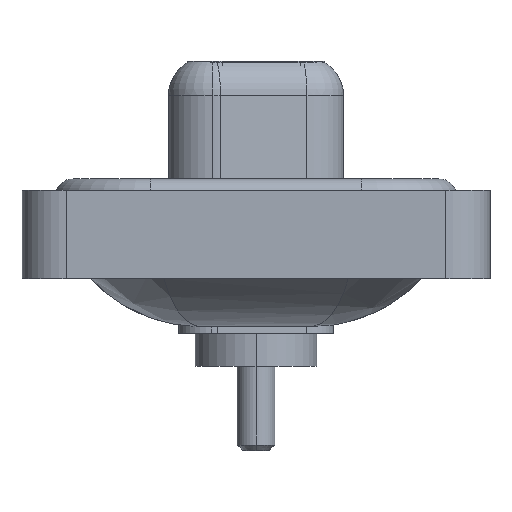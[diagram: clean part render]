
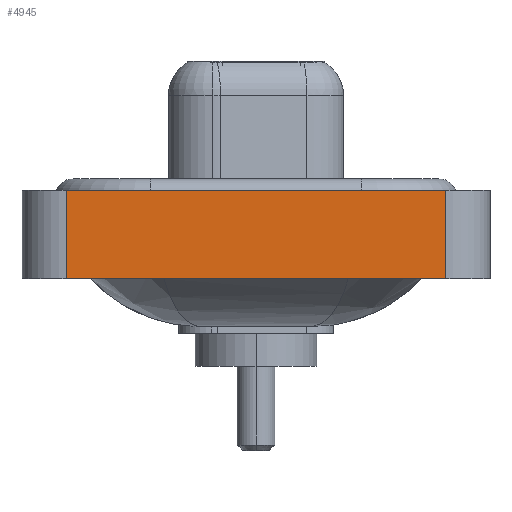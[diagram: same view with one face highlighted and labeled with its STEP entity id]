
A CAD part, left-side view. The second image highlights one B-rep face of the part: STEP entity #4945.
In plain terms, the highlighted planar face has unit normal (-1, 0, 0).
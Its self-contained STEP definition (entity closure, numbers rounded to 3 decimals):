
#272 = ORIENTED_EDGE ( 'NONE', *, *, #8053, .T. ) ;
#815 = VECTOR ( 'NONE', #5767, 1000. ) ;
#1399 = CARTESIAN_POINT ( 'NONE',  ( -7.25, -8.55, -3.6 ) ) ;
#1463 = CARTESIAN_POINT ( 'NONE',  ( -7.25, -8.55, -3.6 ) ) ;
#2579 = FACE_OUTER_BOUND ( 'NONE', #5798, .T. ) ;
#2934 = VERTEX_POINT ( 'NONE', #13214 ) ;
#4371 = AXIS2_PLACEMENT_3D ( 'NONE', #1463, #12279, #5270 ) ;
#4435 = EDGE_CURVE ( 'NONE', #11195, #14552, #9726, .T. ) ;
#4510 = DIRECTION ( 'NONE',  ( 0., -1., 0. ) ) ;
#4674 = LINE ( 'NONE', #14365, #11908 ) ;
#4945 = ADVANCED_FACE ( 'NONE', ( #2579 ), #7496, .T. ) ;
#5270 = DIRECTION ( 'NONE',  ( 0., 0., 1. ) ) ;
#5298 = ORIENTED_EDGE ( 'NONE', *, *, #14034, .F. ) ;
#5333 = ORIENTED_EDGE ( 'NONE', *, *, #4435, .F. ) ;
#5767 = DIRECTION ( 'NONE',  ( 0., 0., 1. ) ) ;
#5798 = EDGE_LOOP ( 'NONE', ( #272, #5298, #5333, #13059 ) ) ;
#6933 = LINE ( 'NONE', #9223, #7420 ) ;
#7004 = CARTESIAN_POINT ( 'NONE',  ( -7.25, 8.55, -3.6 ) ) ;
#7420 = VECTOR ( 'NONE', #14178, 1000. ) ;
#7496 = PLANE ( 'NONE',  #4371 ) ;
#8053 = EDGE_CURVE ( 'NONE', #9758, #2934, #6933, .T. ) ;
#9223 = CARTESIAN_POINT ( 'NONE',  ( -7.25, -8.55, -3.6 ) ) ;
#9413 = CARTESIAN_POINT ( 'NONE',  ( -7.25, 8.55, -3.6 ) ) ;
#9726 = LINE ( 'NONE', #9413, #815 ) ;
#9758 = VERTEX_POINT ( 'NONE', #1399 ) ;
#10093 = CARTESIAN_POINT ( 'NONE',  ( -7.25, 8.55, 0.4 ) ) ;
#11195 = VERTEX_POINT ( 'NONE', #7004 ) ;
#11714 = EDGE_CURVE ( 'NONE', #11195, #9758, #4674, .T. ) ;
#11908 = VECTOR ( 'NONE', #4510, 1000. ) ;
#12279 = DIRECTION ( 'NONE',  ( -1., 0., 0. ) ) ;
#12940 = DIRECTION ( 'NONE',  ( 0., -1., 0. ) ) ;
#13059 = ORIENTED_EDGE ( 'NONE', *, *, #11714, .T. ) ;
#13174 = CARTESIAN_POINT ( 'NONE',  ( -7.25, -8.55, 0.4 ) ) ;
#13214 = CARTESIAN_POINT ( 'NONE',  ( -7.25, -8.55, 0.4 ) ) ;
#14034 = EDGE_CURVE ( 'NONE', #14552, #2934, #14355, .T. ) ;
#14178 = DIRECTION ( 'NONE',  ( 0., 0., 1. ) ) ;
#14206 = VECTOR ( 'NONE', #12940, 1000. ) ;
#14355 = LINE ( 'NONE', #13174, #14206 ) ;
#14365 = CARTESIAN_POINT ( 'NONE',  ( -7.25, -8.55, -3.6 ) ) ;
#14552 = VERTEX_POINT ( 'NONE', #10093 ) ;
